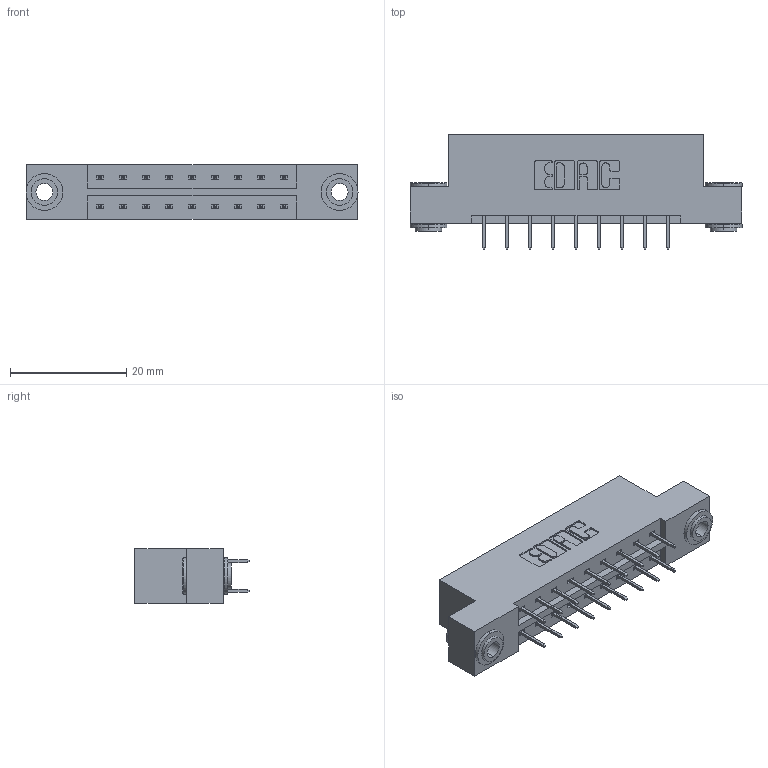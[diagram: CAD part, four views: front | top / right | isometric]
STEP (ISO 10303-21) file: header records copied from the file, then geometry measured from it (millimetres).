
FILE_DESCRIPTION (( 'STEP AP203' ), '1' );
FILE_NAME ('333-018-524-203.STEP', '2019-08-09T13:09:20', ( '' ), ( '' ), 'SwSTEP 2.0', 'SolidWorks 2016', '' );
FILE_SCHEMA (( 'CONFIG_CONTROL_DESIGN' ));
Length unit declared in the file: inch
Products named in the file (4): 333 Part_Flush - .156 Dia - TH; 333-018-524-203; 345-292-001_345-293-124; 345-250-002_345-250-002-102
Assembly tree (21 placements, depth 2):
  333-018-524-203
    333 Part_Flush - .156 Dia - TH
    345-292-001_345-293-124  x18
    345-250-002_345-250-002-102  x2
Bounding box: 57.2 x 19.69 x 9.4 mm (x, y, z)
Volume: 5523.4 mm3; surface area: 6314.6 mm2
Topology: 21 solids, 21 shells, 1160 faces, 3249 edges, 2090 vertices
Faces by surface type: plane 836, cylinder 316, cone 8
Entity records: 10782 total; most frequent: CARTESIAN_POINT 1801, ORIENTED_EDGE 1730, DIRECTION 1631, EDGE_CURVE 865, VECTOR 717, LINE 717, VERTEX_POINT 570, AXIS2_PLACEMENT_3D 457
